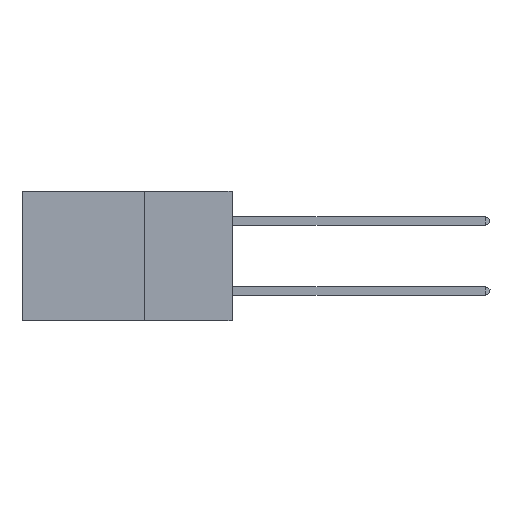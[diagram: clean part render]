
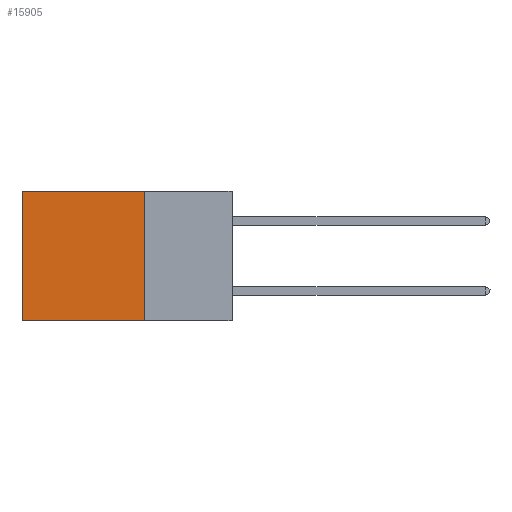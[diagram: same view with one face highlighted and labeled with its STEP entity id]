
A CAD part, left-side view. The second image highlights one B-rep face of the part: STEP entity #15905.
In plain terms, the highlighted planar face has unit normal (-1, 0, 0).
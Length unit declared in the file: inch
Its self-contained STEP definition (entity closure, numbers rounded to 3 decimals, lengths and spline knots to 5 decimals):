
#177 = CARTESIAN_POINT ( 'NONE',  ( 0.2875, 0.25, -0.37 ) ) ;
#910 = CARTESIAN_POINT ( 'NONE',  ( 0.2875, 0.25, -0.37 ) ) ;
#1102 = EDGE_CURVE ( 'NONE', #11551, #9936, #11524, .T. ) ;
#1366 = VERTEX_POINT ( 'NONE', #177 ) ;
#3085 = CARTESIAN_POINT ( 'NONE',  ( 0.2875, 0.25, 0. ) ) ;
#3828 = CARTESIAN_POINT ( 'NONE',  ( 0.2875, 0.25, 0. ) ) ;
#4395 = CARTESIAN_POINT ( 'NONE',  ( 0.2875, 0.25, 0. ) ) ;
#4692 = DIRECTION ( 'NONE',  ( 0., 1., 0. ) ) ;
#5095 = PLANE ( 'NONE',  #5441 ) ;
#5441 = AXIS2_PLACEMENT_3D ( 'NONE', #3828, #14723, #6802 ) ;
#5621 = EDGE_LOOP ( 'NONE', ( #7465, #11678, #14236, #14443 ) ) ;
#6574 = VECTOR ( 'NONE', #4692, 39.37008 ) ;
#6629 = FACE_OUTER_BOUND ( 'NONE', #5621, .T. ) ;
#6802 = DIRECTION ( 'NONE',  ( 0., 0., -1. ) ) ;
#7465 = ORIENTED_EDGE ( 'NONE', *, *, #17529, .T. ) ;
#7598 = CARTESIAN_POINT ( 'NONE',  ( 0.2875, 0.6, 0. ) ) ;
#8441 = LINE ( 'NONE', #4395, #12615 ) ;
#9928 = VECTOR ( 'NONE', #10432, 39.37008 ) ;
#9936 = VERTEX_POINT ( 'NONE', #12339 ) ;
#10432 = DIRECTION ( 'NONE',  ( 0., 1., 0. ) ) ;
#11506 = DIRECTION ( 'NONE',  ( 0., 0., -1. ) ) ;
#11524 = LINE ( 'NONE', #11692, #9928 ) ;
#11551 = VERTEX_POINT ( 'NONE', #3085 ) ;
#11678 = ORIENTED_EDGE ( 'NONE', *, *, #16016, .F. ) ;
#11692 = CARTESIAN_POINT ( 'NONE',  ( 0.2875, 0.25, 0. ) ) ;
#11749 = VECTOR ( 'NONE', #15801, 39.37008 ) ;
#12339 = CARTESIAN_POINT ( 'NONE',  ( 0.2875, 0.6, 0. ) ) ;
#12615 = VECTOR ( 'NONE', #11506, 39.37008 ) ;
#12809 = CARTESIAN_POINT ( 'NONE',  ( 0.2875, 0.6, -0.37 ) ) ;
#12978 = VERTEX_POINT ( 'NONE', #12809 ) ;
#14236 = ORIENTED_EDGE ( 'NONE', *, *, #15164, .F. ) ;
#14417 = LINE ( 'NONE', #910, #6574 ) ;
#14443 = ORIENTED_EDGE ( 'NONE', *, *, #1102, .T. ) ;
#14721 = LINE ( 'NONE', #7598, #11749 ) ;
#14723 = DIRECTION ( 'NONE',  ( 1., 0., 0. ) ) ;
#15164 = EDGE_CURVE ( 'NONE', #11551, #1366, #8441, .T. ) ;
#15801 = DIRECTION ( 'NONE',  ( 0., 0., -1. ) ) ;
#15905 = ADVANCED_FACE ( 'NONE', ( #6629 ), #5095, .F. ) ;
#16016 = EDGE_CURVE ( 'NONE', #1366, #12978, #14417, .T. ) ;
#17529 = EDGE_CURVE ( 'NONE', #9936, #12978, #14721, .T. ) ;
